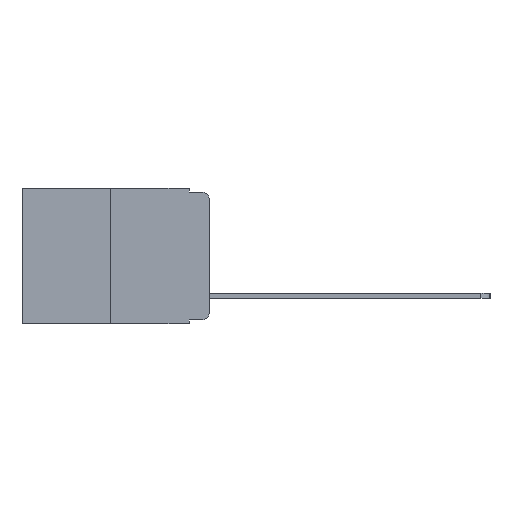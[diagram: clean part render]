
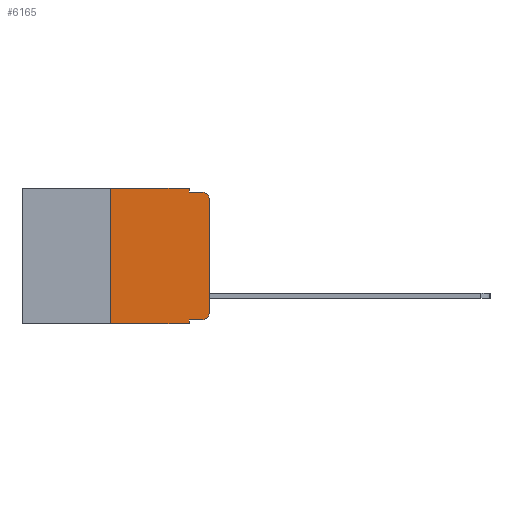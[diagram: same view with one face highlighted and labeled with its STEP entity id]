
A CAD part, left-side view. The second image highlights one B-rep face of the part: STEP entity #6165.
In plain terms, the highlighted planar face has unit normal (-1, 0, 0).
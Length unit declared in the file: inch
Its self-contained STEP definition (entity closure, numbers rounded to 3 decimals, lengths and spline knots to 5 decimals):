
#165 = ORIENTED_EDGE ( 'NONE', *, *, #12262, .F. ) ;
#421 = CARTESIAN_POINT ( 'NONE',  ( 0., 0.473, 0. ) ) ;
#1309 = EDGE_LOOP ( 'NONE', ( #18000, #15315, #165, #15617, #17894, #6023, #20028, #11976, #9155, #13429 ) ) ;
#1401 = DIRECTION ( 'NONE',  ( 0., 0., 1. ) ) ;
#1608 = CARTESIAN_POINT ( 'NONE',  ( 0., 0.051, 0. ) ) ;
#1647 = LINE ( 'NONE', #2126, #14439 ) ;
#2051 = EDGE_CURVE ( 'NONE', #3906, #17399, #14426, .T. ) ;
#2056 = LINE ( 'NONE', #4969, #10416 ) ;
#2104 = DIRECTION ( 'NONE',  ( 1., 0., 0. ) ) ;
#2126 = CARTESIAN_POINT ( 'NONE',  ( 0., 0.051, 0. ) ) ;
#3192 = AXIS2_PLACEMENT_3D ( 'NONE', #421, #2104, #13784 ) ;
#3323 = VECTOR ( 'NONE', #17443, 39.37008 ) ;
#3416 = AXIS2_PLACEMENT_3D ( 'NONE', #12992, #13229, #13210 ) ;
#3862 = LINE ( 'NONE', #15777, #3323 ) ;
#3906 = VERTEX_POINT ( 'NONE', #19461 ) ;
#4165 = CARTESIAN_POINT ( 'NONE',  ( 0., 0.051, -0.333 ) ) ;
#4475 = CARTESIAN_POINT ( 'NONE',  ( 0., 0., 0. ) ) ;
#4618 = DIRECTION ( 'NONE',  ( 0., -1., 0. ) ) ;
#4757 = FACE_OUTER_BOUND ( 'NONE', #1309, .T. ) ;
#4969 = CARTESIAN_POINT ( 'NONE',  ( 0., 0.051, -0.01 ) ) ;
#5167 = EDGE_CURVE ( 'NONE', #6801, #9052, #15044, .T. ) ;
#5263 = VERTEX_POINT ( 'NONE', #1608 ) ;
#5313 = EDGE_CURVE ( 'NONE', #15806, #14833, #7515, .T. ) ;
#5614 = VECTOR ( 'NONE', #4618, 39.37008 ) ;
#5633 = VECTOR ( 'NONE', #20123, 39.37008 ) ;
#6023 = ORIENTED_EDGE ( 'NONE', *, *, #5167, .F. ) ;
#6165 = ADVANCED_FACE ( 'NONE', ( #4757 ), #15360, .F. ) ;
#6801 = VERTEX_POINT ( 'NONE', #13830 ) ;
#7515 = CIRCLE ( 'NONE', #11133, 0.02 ) ;
#7814 = VERTEX_POINT ( 'NONE', #11756 ) ;
#7960 = CARTESIAN_POINT ( 'NONE',  ( 0., 0.25, 0. ) ) ;
#8098 = EDGE_CURVE ( 'NONE', #13807, #3906, #3862, .T. ) ;
#8502 = CARTESIAN_POINT ( 'NONE',  ( 0., 0.02, -0.03 ) ) ;
#9052 = VERTEX_POINT ( 'NONE', #7960 ) ;
#9155 = ORIENTED_EDGE ( 'NONE', *, *, #8098, .T. ) ;
#9658 = VECTOR ( 'NONE', #16085, 39.37008 ) ;
#9947 = EDGE_CURVE ( 'NONE', #9052, #5263, #13944, .T. ) ;
#10006 = LINE ( 'NONE', #21104, #5614 ) ;
#10045 = VECTOR ( 'NONE', #19589, 39.37008 ) ;
#10150 = DIRECTION ( 'NONE',  ( 0., 0., -1. ) ) ;
#10313 = EDGE_CURVE ( 'NONE', #6801, #7814, #10006, .T. ) ;
#10416 = VECTOR ( 'NONE', #11642, 39.37008 ) ;
#10450 = DIRECTION ( 'NONE',  ( 0., 0., -1. ) ) ;
#10611 = CARTESIAN_POINT ( 'NONE',  ( 0., 0., -0.313 ) ) ;
#10619 = VECTOR ( 'NONE', #1401, 39.37008 ) ;
#11133 = AXIS2_PLACEMENT_3D ( 'NONE', #8502, #20045, #10150 ) ;
#11392 = CARTESIAN_POINT ( 'NONE',  ( 0., 0.25, 0. ) ) ;
#11642 = DIRECTION ( 'NONE',  ( 0., -1., 0. ) ) ;
#11756 = CARTESIAN_POINT ( 'NONE',  ( 0., 0.051, -0.343 ) ) ;
#11976 = ORIENTED_EDGE ( 'NONE', *, *, #16268, .F. ) ;
#12262 = EDGE_CURVE ( 'NONE', #14385, #14833, #2056, .T. ) ;
#12992 = CARTESIAN_POINT ( 'NONE',  ( 0., 0.02, -0.313 ) ) ;
#13210 = DIRECTION ( 'NONE',  ( 0., 0., -1. ) ) ;
#13229 = DIRECTION ( 'NONE',  ( -1., 0., 0. ) ) ;
#13271 = CARTESIAN_POINT ( 'NONE',  ( 0., 0.02, -0.01 ) ) ;
#13429 = ORIENTED_EDGE ( 'NONE', *, *, #2051, .T. ) ;
#13784 = DIRECTION ( 'NONE',  ( 0., 0., -1. ) ) ;
#13807 = VERTEX_POINT ( 'NONE', #4165 ) ;
#13830 = CARTESIAN_POINT ( 'NONE',  ( 0., 0.25, -0.343 ) ) ;
#13944 = LINE ( 'NONE', #15232, #5633 ) ;
#14087 = LINE ( 'NONE', #4475, #9658 ) ;
#14385 = VERTEX_POINT ( 'NONE', #18683 ) ;
#14426 = CIRCLE ( 'NONE', #3416, 0.02 ) ;
#14439 = VECTOR ( 'NONE', #10450, 39.37008 ) ;
#14833 = VERTEX_POINT ( 'NONE', #13271 ) ;
#15044 = LINE ( 'NONE', #11392, #10619 ) ;
#15232 = CARTESIAN_POINT ( 'NONE',  ( 0., 0.473, 0. ) ) ;
#15286 = EDGE_CURVE ( 'NONE', #5263, #14385, #18852, .T. ) ;
#15315 = ORIENTED_EDGE ( 'NONE', *, *, #5313, .T. ) ;
#15360 = PLANE ( 'NONE',  #3192 ) ;
#15617 = ORIENTED_EDGE ( 'NONE', *, *, #15286, .F. ) ;
#15777 = CARTESIAN_POINT ( 'NONE',  ( 0., 0.051, -0.333 ) ) ;
#15806 = VERTEX_POINT ( 'NONE', #20843 ) ;
#16085 = DIRECTION ( 'NONE',  ( 0., 0., 1. ) ) ;
#16268 = EDGE_CURVE ( 'NONE', #13807, #7814, #1647, .T. ) ;
#17399 = VERTEX_POINT ( 'NONE', #10611 ) ;
#17443 = DIRECTION ( 'NONE',  ( 0., -1., 0. ) ) ;
#17894 = ORIENTED_EDGE ( 'NONE', *, *, #9947, .F. ) ;
#17922 = CARTESIAN_POINT ( 'NONE',  ( 0., 0.051, 0. ) ) ;
#18000 = ORIENTED_EDGE ( 'NONE', *, *, #18178, .T. ) ;
#18178 = EDGE_CURVE ( 'NONE', #17399, #15806, #14087, .T. ) ;
#18683 = CARTESIAN_POINT ( 'NONE',  ( 0., 0.051, -0.01 ) ) ;
#18852 = LINE ( 'NONE', #17922, #10045 ) ;
#19461 = CARTESIAN_POINT ( 'NONE',  ( 0., 0.02, -0.333 ) ) ;
#19589 = DIRECTION ( 'NONE',  ( 0., 0., -1. ) ) ;
#20028 = ORIENTED_EDGE ( 'NONE', *, *, #10313, .T. ) ;
#20045 = DIRECTION ( 'NONE',  ( -1., 0., 0. ) ) ;
#20123 = DIRECTION ( 'NONE',  ( 0., -1., 0. ) ) ;
#20843 = CARTESIAN_POINT ( 'NONE',  ( 0., 0., -0.03 ) ) ;
#21104 = CARTESIAN_POINT ( 'NONE',  ( 0., 0.473, -0.343 ) ) ;
